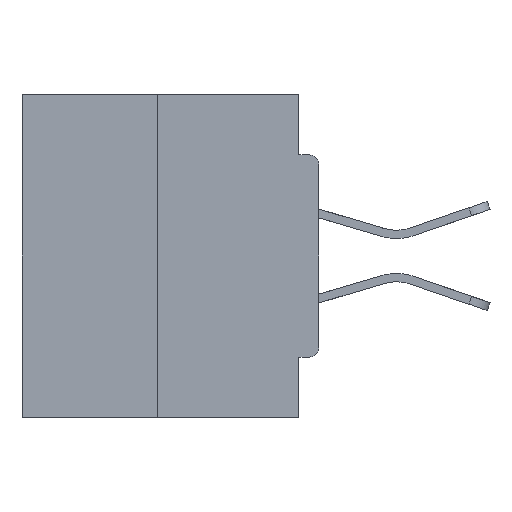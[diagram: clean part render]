
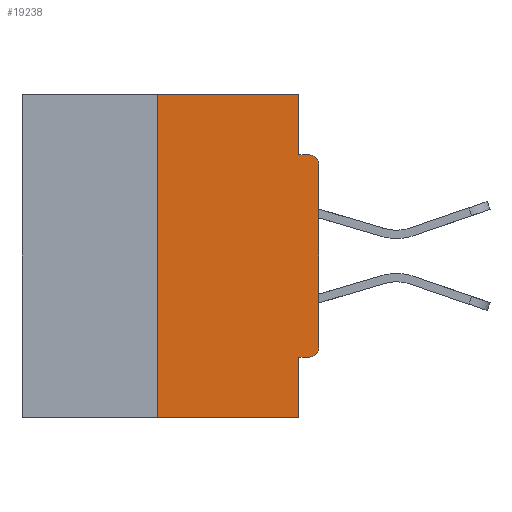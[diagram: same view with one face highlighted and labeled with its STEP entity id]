
A CAD part, left-side view. The second image highlights one B-rep face of the part: STEP entity #19238.
In plain terms, the highlighted planar face has unit normal (-1, 0, 0).
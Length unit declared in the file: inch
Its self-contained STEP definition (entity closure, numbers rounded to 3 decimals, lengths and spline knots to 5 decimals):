
#281 = DIRECTION ( 'NONE',  ( 0., 0., -1. ) ) ;
#436 = CARTESIAN_POINT ( 'NONE',  ( 0., 0.015, -0.0935 ) ) ;
#498 = DIRECTION ( 'NONE',  ( 0., -1., 0. ) ) ;
#816 = PLANE ( 'NONE',  #12737 ) ;
#946 = CARTESIAN_POINT ( 'NONE',  ( 0., 0., -0.4065 ) ) ;
#995 = VERTEX_POINT ( 'NONE', #23364 ) ;
#1347 = ORIENTED_EDGE ( 'NONE', *, *, #15613, .F. ) ;
#1799 = CARTESIAN_POINT ( 'NONE',  ( 0., 0.25, -0.5 ) ) ;
#1911 = EDGE_CURVE ( 'NONE', #8000, #3567, #23783, .T. ) ;
#2573 = ORIENTED_EDGE ( 'NONE', *, *, #12676, .F. ) ;
#2855 = LINE ( 'NONE', #15684, #18690 ) ;
#2985 = EDGE_CURVE ( 'NONE', #3567, #4466, #22684, .T. ) ;
#3199 = DIRECTION ( 'NONE',  ( 0., 0., -1. ) ) ;
#3567 = VERTEX_POINT ( 'NONE', #19833 ) ;
#3856 = CARTESIAN_POINT ( 'NONE',  ( 0., 0.46, 0. ) ) ;
#4466 = VERTEX_POINT ( 'NONE', #436 ) ;
#4503 = ORIENTED_EDGE ( 'NONE', *, *, #5830, .F. ) ;
#5145 = CARTESIAN_POINT ( 'NONE',  ( 0., 0.031, 0. ) ) ;
#5830 = EDGE_CURVE ( 'NONE', #8429, #31656, #21016, .T. ) ;
#6106 = VERTEX_POINT ( 'NONE', #7455 ) ;
#6159 = LINE ( 'NONE', #28590, #26073 ) ;
#7455 = CARTESIAN_POINT ( 'NONE',  ( 0., 0.25, 0. ) ) ;
#8000 = VERTEX_POINT ( 'NONE', #29651 ) ;
#8015 = ORIENTED_EDGE ( 'NONE', *, *, #30672, .F. ) ;
#8429 = VERTEX_POINT ( 'NONE', #21925 ) ;
#8543 = DIRECTION ( 'NONE',  ( 0., 0., 1. ) ) ;
#10004 = CARTESIAN_POINT ( 'NONE',  ( 0., 0.031, 0. ) ) ;
#10008 = ORIENTED_EDGE ( 'NONE', *, *, #31433, .F. ) ;
#10021 = EDGE_CURVE ( 'NONE', #22332, #31656, #31781, .T. ) ;
#10310 = CARTESIAN_POINT ( 'NONE',  ( 0., 0.015, -0.3915 ) ) ;
#10478 = VECTOR ( 'NONE', #19375, 39.37008 ) ;
#12268 = VECTOR ( 'NONE', #32254, 39.37008 ) ;
#12676 = EDGE_CURVE ( 'NONE', #19964, #4466, #6159, .T. ) ;
#12737 = AXIS2_PLACEMENT_3D ( 'NONE', #3856, #28953, #14162 ) ;
#13432 = ORIENTED_EDGE ( 'NONE', *, *, #2985, .T. ) ;
#14162 = DIRECTION ( 'NONE',  ( 0., 0., -1. ) ) ;
#15613 = EDGE_CURVE ( 'NONE', #25779, #19964, #32467, .T. ) ;
#15684 = CARTESIAN_POINT ( 'NONE',  ( 0., 0.46, 0. ) ) ;
#16234 = EDGE_LOOP ( 'NONE', ( #10008, #23168, #23244, #4503, #8015, #24775, #27160, #13432, #2573, #1347 ) ) ;
#16336 = CARTESIAN_POINT ( 'NONE',  ( 0., 0.015, -0.1085 ) ) ;
#16515 = FACE_OUTER_BOUND ( 'NONE', #16234, .T. ) ;
#16737 = VECTOR ( 'NONE', #8543, 39.37008 ) ;
#16806 = LINE ( 'NONE', #946, #12268 ) ;
#16984 = CIRCLE ( 'NONE', #30375, 0.015 ) ;
#17344 = LINE ( 'NONE', #27552, #10478 ) ;
#18178 = DIRECTION ( 'NONE',  ( -1., 0., 0. ) ) ;
#18402 = CARTESIAN_POINT ( 'NONE',  ( 0., 0., 0. ) ) ;
#18690 = VECTOR ( 'NONE', #498, 39.37008 ) ;
#19206 = CARTESIAN_POINT ( 'NONE',  ( 0., 0.031, -0.5 ) ) ;
#19238 = ADVANCED_FACE ( 'NONE', ( #16515 ), #816, .F. ) ;
#19375 = DIRECTION ( 'NONE',  ( 0., 0., 1. ) ) ;
#19546 = DIRECTION ( 'NONE',  ( 0., 0., -1. ) ) ;
#19833 = CARTESIAN_POINT ( 'NONE',  ( 0., 0., -0.1085 ) ) ;
#19964 = VERTEX_POINT ( 'NONE', #31054 ) ;
#20514 = AXIS2_PLACEMENT_3D ( 'NONE', #16336, #28956, #3199 ) ;
#20760 = EDGE_CURVE ( 'NONE', #995, #8000, #16984, .T. ) ;
#21016 = LINE ( 'NONE', #21678, #25635 ) ;
#21541 = CARTESIAN_POINT ( 'NONE',  ( 0., 0.46, -0.5 ) ) ;
#21678 = CARTESIAN_POINT ( 'NONE',  ( 0., 0.031, -0.5 ) ) ;
#21714 = DIRECTION ( 'NONE',  ( 0., -1., 0. ) ) ;
#21925 = CARTESIAN_POINT ( 'NONE',  ( 0., 0.031, -0.4065 ) ) ;
#22332 = VERTEX_POINT ( 'NONE', #1799 ) ;
#22684 = CIRCLE ( 'NONE', #20514, 0.015 ) ;
#23088 = VECTOR ( 'NONE', #28932, 39.37008 ) ;
#23168 = ORIENTED_EDGE ( 'NONE', *, *, #25668, .F. ) ;
#23244 = ORIENTED_EDGE ( 'NONE', *, *, #10021, .T. ) ;
#23364 = CARTESIAN_POINT ( 'NONE',  ( 0., 0.015, -0.4065 ) ) ;
#23783 = LINE ( 'NONE', #18402, #16737 ) ;
#24775 = ORIENTED_EDGE ( 'NONE', *, *, #20760, .T. ) ;
#25635 = VECTOR ( 'NONE', #26036, 39.37008 ) ;
#25668 = EDGE_CURVE ( 'NONE', #22332, #6106, #17344, .T. ) ;
#25779 = VERTEX_POINT ( 'NONE', #5145 ) ;
#26036 = DIRECTION ( 'NONE',  ( 0., 0., -1. ) ) ;
#26073 = VECTOR ( 'NONE', #21714, 39.37008 ) ;
#27160 = ORIENTED_EDGE ( 'NONE', *, *, #1911, .T. ) ;
#27213 = VECTOR ( 'NONE', #19546, 39.37008 ) ;
#27552 = CARTESIAN_POINT ( 'NONE',  ( 0., 0.25, 0. ) ) ;
#28590 = CARTESIAN_POINT ( 'NONE',  ( 0., 0., -0.0935 ) ) ;
#28932 = DIRECTION ( 'NONE',  ( 0., -1., 0. ) ) ;
#28953 = DIRECTION ( 'NONE',  ( 1., 0., 0. ) ) ;
#28956 = DIRECTION ( 'NONE',  ( -1., 0., 0. ) ) ;
#29651 = CARTESIAN_POINT ( 'NONE',  ( 0., 0., -0.3915 ) ) ;
#30375 = AXIS2_PLACEMENT_3D ( 'NONE', #10310, #18178, #281 ) ;
#30672 = EDGE_CURVE ( 'NONE', #995, #8429, #16806, .T. ) ;
#31054 = CARTESIAN_POINT ( 'NONE',  ( 0., 0.031, -0.0935 ) ) ;
#31433 = EDGE_CURVE ( 'NONE', #6106, #25779, #2855, .T. ) ;
#31656 = VERTEX_POINT ( 'NONE', #19206 ) ;
#31781 = LINE ( 'NONE', #21541, #23088 ) ;
#32254 = DIRECTION ( 'NONE',  ( 0., 1., 0. ) ) ;
#32467 = LINE ( 'NONE', #10004, #27213 ) ;
